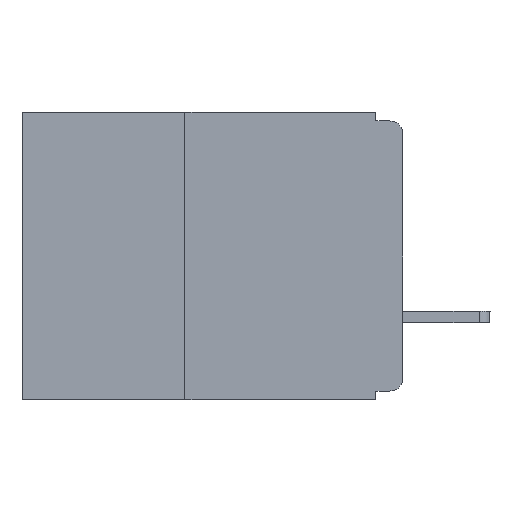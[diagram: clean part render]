
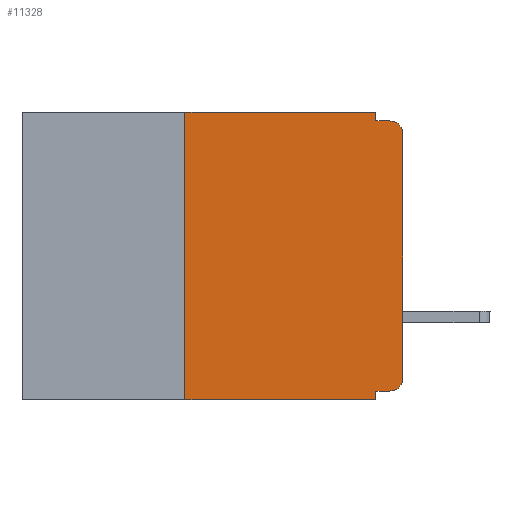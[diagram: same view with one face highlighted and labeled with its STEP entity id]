
A CAD part, left-side view. The second image highlights one B-rep face of the part: STEP entity #11328.
In plain terms, the highlighted planar face has unit normal (-1, 0, 0).
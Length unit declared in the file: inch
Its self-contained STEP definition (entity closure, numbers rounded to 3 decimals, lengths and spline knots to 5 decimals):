
#192 = EDGE_CURVE ( 'NONE', #12086, #9920, #6970, .T. ) ;
#420 = CARTESIAN_POINT ( 'NONE',  ( 0., 0., -0.025 ) ) ;
#450 = VECTOR ( 'NONE', #2744, 39.37008 ) ;
#504 = CARTESIAN_POINT ( 'NONE',  ( 0., 0., -0.305 ) ) ;
#548 = ORIENTED_EDGE ( 'NONE', *, *, #4558, .T. ) ;
#569 = VECTOR ( 'NONE', #2653, 39.37008 ) ;
#893 = LINE ( 'NONE', #3536, #569 ) ;
#898 = PLANE ( 'NONE',  #6817 ) ;
#913 = CARTESIAN_POINT ( 'NONE',  ( 0., 0.437, -0.33 ) ) ;
#1042 = ORIENTED_EDGE ( 'NONE', *, *, #7388, .F. ) ;
#1099 = DIRECTION ( 'NONE',  ( 0., 0., -1. ) ) ;
#1119 = DIRECTION ( 'NONE',  ( 0., 0., -1. ) ) ;
#1275 = EDGE_LOOP ( 'NONE', ( #548, #7373, #8014, #9895, #1042, #9966, #3880, #12922, #3466, #12260 ) ) ;
#1499 = EDGE_CURVE ( 'NONE', #12561, #9957, #3146, .T. ) ;
#1700 = DIRECTION ( 'NONE',  ( 0., 0., -1. ) ) ;
#1745 = LINE ( 'NONE', #6541, #450 ) ;
#1760 = CARTESIAN_POINT ( 'NONE',  ( 0., 0.25, 0. ) ) ;
#1817 = DIRECTION ( 'NONE',  ( 0., -1., 0. ) ) ;
#1886 = CARTESIAN_POINT ( 'NONE',  ( 0., 0.031, -0.33 ) ) ;
#1984 = EDGE_CURVE ( 'NONE', #11836, #4530, #3449, .T. ) ;
#2184 = DIRECTION ( 'NONE',  ( 0., 0., -1. ) ) ;
#2504 = VECTOR ( 'NONE', #10221, 39.37008 ) ;
#2545 = AXIS2_PLACEMENT_3D ( 'NONE', #9400, #3294, #1099 ) ;
#2653 = DIRECTION ( 'NONE',  ( 0., -1., 0. ) ) ;
#2728 = LINE ( 'NONE', #8295, #8945 ) ;
#2744 = DIRECTION ( 'NONE',  ( 0., 0., 1. ) ) ;
#2823 = FACE_OUTER_BOUND ( 'NONE', #1275, .T. ) ;
#3063 = CARTESIAN_POINT ( 'NONE',  ( 0., 0.25, -0.33 ) ) ;
#3093 = DIRECTION ( 'NONE',  ( 1., 0., 0. ) ) ;
#3146 = LINE ( 'NONE', #913, #2504 ) ;
#3294 = DIRECTION ( 'NONE',  ( -1., 0., 0. ) ) ;
#3449 = CIRCLE ( 'NONE', #11133, 0.015 ) ;
#3466 = ORIENTED_EDGE ( 'NONE', *, *, #11655, .F. ) ;
#3536 = CARTESIAN_POINT ( 'NONE',  ( 0., 0.437, 0. ) ) ;
#3880 = ORIENTED_EDGE ( 'NONE', *, *, #1499, .T. ) ;
#4530 = VERTEX_POINT ( 'NONE', #504 ) ;
#4558 = EDGE_CURVE ( 'NONE', #4530, #10582, #1745, .T. ) ;
#5006 = CARTESIAN_POINT ( 'NONE',  ( 0., 0., -0.01 ) ) ;
#5340 = VECTOR ( 'NONE', #9045, 39.37008 ) ;
#5481 = CARTESIAN_POINT ( 'NONE',  ( 0., 0.25, -0.33 ) ) ;
#5553 = CIRCLE ( 'NONE', #2545, 0.015 ) ;
#5697 = VECTOR ( 'NONE', #1817, 39.37008 ) ;
#6154 = DIRECTION ( 'NONE',  ( 0., 0., 1. ) ) ;
#6541 = CARTESIAN_POINT ( 'NONE',  ( 0., 0., 0. ) ) ;
#6578 = EDGE_CURVE ( 'NONE', #8289, #12086, #2728, .T. ) ;
#6817 = AXIS2_PLACEMENT_3D ( 'NONE', #7121, #3093, #11269 ) ;
#6970 = LINE ( 'NONE', #5006, #5697 ) ;
#6987 = CARTESIAN_POINT ( 'NONE',  ( 0., 0.031, -0.33 ) ) ;
#7121 = CARTESIAN_POINT ( 'NONE',  ( 0., 0.437, 0. ) ) ;
#7373 = ORIENTED_EDGE ( 'NONE', *, *, #10874, .T. ) ;
#7388 = EDGE_CURVE ( 'NONE', #11289, #8289, #893, .T. ) ;
#7885 = LINE ( 'NONE', #8010, #5340 ) ;
#8010 = CARTESIAN_POINT ( 'NONE',  ( 0., 0., -0.32 ) ) ;
#8014 = ORIENTED_EDGE ( 'NONE', *, *, #192, .F. ) ;
#8289 = VERTEX_POINT ( 'NONE', #8546 ) ;
#8295 = CARTESIAN_POINT ( 'NONE',  ( 0., 0.031, 0. ) ) ;
#8546 = CARTESIAN_POINT ( 'NONE',  ( 0., 0.031, 0. ) ) ;
#8945 = VECTOR ( 'NONE', #2184, 39.37008 ) ;
#9045 = DIRECTION ( 'NONE',  ( 0., 1., 0. ) ) ;
#9068 = CARTESIAN_POINT ( 'NONE',  ( 0., 0.015, -0.01 ) ) ;
#9199 = CARTESIAN_POINT ( 'NONE',  ( 0., 0.015, -0.305 ) ) ;
#9400 = CARTESIAN_POINT ( 'NONE',  ( 0., 0.015, -0.025 ) ) ;
#9895 = ORIENTED_EDGE ( 'NONE', *, *, #6578, .F. ) ;
#9920 = VERTEX_POINT ( 'NONE', #9068 ) ;
#9957 = VERTEX_POINT ( 'NONE', #6987 ) ;
#9966 = ORIENTED_EDGE ( 'NONE', *, *, #12311, .F. ) ;
#10043 = CARTESIAN_POINT ( 'NONE',  ( 0., 0.015, -0.32 ) ) ;
#10201 = DIRECTION ( 'NONE',  ( -1., 0., 0. ) ) ;
#10221 = DIRECTION ( 'NONE',  ( 0., -1., 0. ) ) ;
#10314 = VECTOR ( 'NONE', #1700, 39.37008 ) ;
#10582 = VERTEX_POINT ( 'NONE', #420 ) ;
#10874 = EDGE_CURVE ( 'NONE', #10582, #9920, #5553, .T. ) ;
#10944 = LINE ( 'NONE', #3063, #13004 ) ;
#11133 = AXIS2_PLACEMENT_3D ( 'NONE', #9199, #10201, #1119 ) ;
#11257 = VERTEX_POINT ( 'NONE', #13013 ) ;
#11269 = DIRECTION ( 'NONE',  ( 0., 0., -1. ) ) ;
#11289 = VERTEX_POINT ( 'NONE', #1760 ) ;
#11328 = ADVANCED_FACE ( 'NONE', ( #2823 ), #898, .F. ) ;
#11655 = EDGE_CURVE ( 'NONE', #11836, #11257, #7885, .T. ) ;
#11671 = EDGE_CURVE ( 'NONE', #11257, #9957, #13030, .T. ) ;
#11836 = VERTEX_POINT ( 'NONE', #10043 ) ;
#12086 = VERTEX_POINT ( 'NONE', #12515 ) ;
#12260 = ORIENTED_EDGE ( 'NONE', *, *, #1984, .T. ) ;
#12311 = EDGE_CURVE ( 'NONE', #12561, #11289, #10944, .T. ) ;
#12515 = CARTESIAN_POINT ( 'NONE',  ( 0., 0.031, -0.01 ) ) ;
#12561 = VERTEX_POINT ( 'NONE', #5481 ) ;
#12922 = ORIENTED_EDGE ( 'NONE', *, *, #11671, .F. ) ;
#13004 = VECTOR ( 'NONE', #6154, 39.37008 ) ;
#13013 = CARTESIAN_POINT ( 'NONE',  ( 0., 0.031, -0.32 ) ) ;
#13030 = LINE ( 'NONE', #1886, #10314 ) ;
